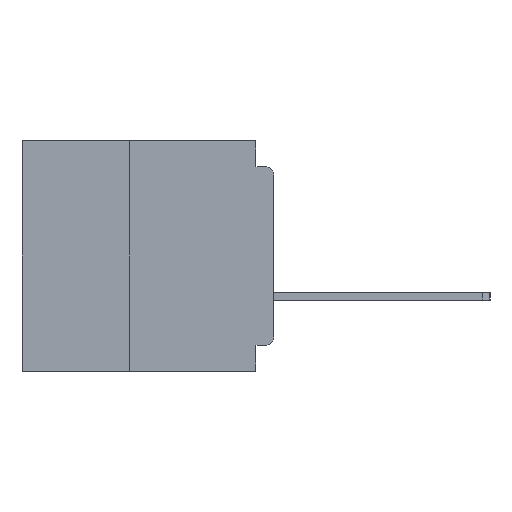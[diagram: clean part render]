
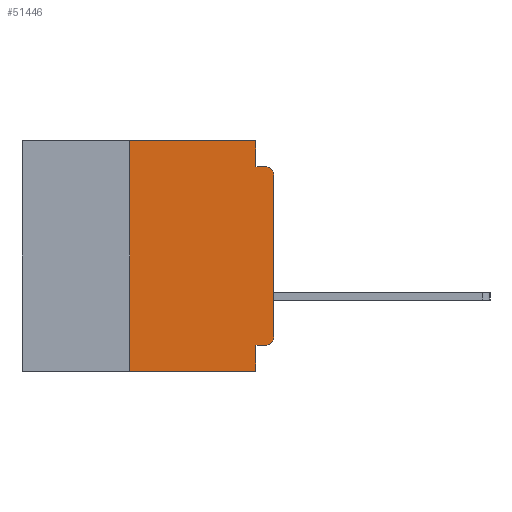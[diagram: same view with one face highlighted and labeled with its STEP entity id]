
A CAD part, left-side view. The second image highlights one B-rep face of the part: STEP entity #51446.
In plain terms, the highlighted planar face has unit normal (-1, 0, 0).
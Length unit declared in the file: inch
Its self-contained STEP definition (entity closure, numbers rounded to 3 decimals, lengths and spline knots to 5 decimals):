
#153 = FACE_OUTER_BOUND ( 'NONE', #14026, .T. ) ;
#730 = EDGE_CURVE ( 'NONE', #28737, #27394, #836, .T. ) ;
#836 = LINE ( 'NONE', #14159, #27034 ) ;
#1958 = EDGE_CURVE ( 'NONE', #6990, #15232, #45787, .T. ) ;
#3212 = CARTESIAN_POINT ( 'NONE',  ( 0., 0.437, 0. ) ) ;
#4133 = CARTESIAN_POINT ( 'NONE',  ( 0., 0.031, -0.355 ) ) ;
#5582 = ORIENTED_EDGE ( 'NONE', *, *, #59781, .F. ) ;
#5728 = LINE ( 'NONE', #22024, #30328 ) ;
#6990 = VERTEX_POINT ( 'NONE', #26731 ) ;
#7189 = AXIS2_PLACEMENT_3D ( 'NONE', #3212, #13134, #47173 ) ;
#8165 = PLANE ( 'NONE',  #7189 ) ;
#8986 = CARTESIAN_POINT ( 'NONE',  ( 0., 0.25, 0. ) ) ;
#9004 = CARTESIAN_POINT ( 'NONE',  ( 0., 0.031, 0. ) ) ;
#9005 = CARTESIAN_POINT ( 'NONE',  ( 0., 0.25, -0.4 ) ) ;
#9928 = LINE ( 'NONE', #20241, #60146 ) ;
#10337 = CIRCLE ( 'NONE', #11037, 0.015 ) ;
#11037 = AXIS2_PLACEMENT_3D ( 'NONE', #41178, #11949, #46035 ) ;
#11949 = DIRECTION ( 'NONE',  ( -1., 0., 0. ) ) ;
#13134 = DIRECTION ( 'NONE',  ( 1., 0., 0. ) ) ;
#13629 = DIRECTION ( 'NONE',  ( 0., 0., -1. ) ) ;
#14026 = EDGE_LOOP ( 'NONE', ( #23141, #17869, #46385, #5582, #19569, #17228, #19658, #22345, #46740, #44199 ) ) ;
#14159 = CARTESIAN_POINT ( 'NONE',  ( 0., 0.031, -0.4 ) ) ;
#14546 = CARTESIAN_POINT ( 'NONE',  ( 0., 0.015, -0.045 ) ) ;
#15232 = VERTEX_POINT ( 'NONE', #26761 ) ;
#15936 = CARTESIAN_POINT ( 'NONE',  ( 0., 0., -0.355 ) ) ;
#17228 = ORIENTED_EDGE ( 'NONE', *, *, #47877, .F. ) ;
#17869 = ORIENTED_EDGE ( 'NONE', *, *, #34002, .T. ) ;
#18106 = EDGE_CURVE ( 'NONE', #44121, #28737, #50356, .T. ) ;
#18987 = EDGE_CURVE ( 'NONE', #44121, #6990, #61621, .T. ) ;
#19569 = ORIENTED_EDGE ( 'NONE', *, *, #21170, .F. ) ;
#19658 = ORIENTED_EDGE ( 'NONE', *, *, #24524, .T. ) ;
#20241 = CARTESIAN_POINT ( 'NONE',  ( 0., 0.25, -0.4 ) ) ;
#21170 = EDGE_CURVE ( 'NONE', #31623, #36889, #34889, .T. ) ;
#21726 = CARTESIAN_POINT ( 'NONE',  ( 0., 0., -0.045 ) ) ;
#21965 = VECTOR ( 'NONE', #40510, 39.37008 ) ;
#22024 = CARTESIAN_POINT ( 'NONE',  ( 0., 0.031, 0. ) ) ;
#22345 = ORIENTED_EDGE ( 'NONE', *, *, #730, .F. ) ;
#23060 = VECTOR ( 'NONE', #55452, 39.37008 ) ;
#23141 = ORIENTED_EDGE ( 'NONE', *, *, #1958, .T. ) ;
#23206 = VERTEX_POINT ( 'NONE', #28243 ) ;
#23985 = VECTOR ( 'NONE', #26770, 39.37008 ) ;
#24524 = EDGE_CURVE ( 'NONE', #56850, #27394, #36855, .T. ) ;
#26731 = CARTESIAN_POINT ( 'NONE',  ( 0., 0., -0.34 ) ) ;
#26761 = CARTESIAN_POINT ( 'NONE',  ( 0., 0., -0.06 ) ) ;
#26770 = DIRECTION ( 'NONE',  ( 0., -1., 0. ) ) ;
#27034 = VECTOR ( 'NONE', #13629, 39.37008 ) ;
#27394 = VERTEX_POINT ( 'NONE', #42565 ) ;
#27434 = CARTESIAN_POINT ( 'NONE',  ( 0., 0.015, -0.34 ) ) ;
#28243 = CARTESIAN_POINT ( 'NONE',  ( 0., 0.031, -0.045 ) ) ;
#28737 = VERTEX_POINT ( 'NONE', #4133 ) ;
#30328 = VECTOR ( 'NONE', #46199, 39.37008 ) ;
#31623 = VERTEX_POINT ( 'NONE', #8986 ) ;
#32284 = DIRECTION ( 'NONE',  ( 0., 0., -1. ) ) ;
#34002 = EDGE_CURVE ( 'NONE', #15232, #50399, #10337, .T. ) ;
#34889 = LINE ( 'NONE', #59780, #21965 ) ;
#36620 = EDGE_CURVE ( 'NONE', #23206, #50399, #61707, .T. ) ;
#36855 = LINE ( 'NONE', #60603, #23985 ) ;
#36889 = VERTEX_POINT ( 'NONE', #9004 ) ;
#37510 = VECTOR ( 'NONE', #49913, 39.37008 ) ;
#40510 = DIRECTION ( 'NONE',  ( 0., -1., 0. ) ) ;
#41178 = CARTESIAN_POINT ( 'NONE',  ( 0., 0.015, -0.06 ) ) ;
#42565 = CARTESIAN_POINT ( 'NONE',  ( 0., 0.031, -0.4 ) ) ;
#44121 = VERTEX_POINT ( 'NONE', #45968 ) ;
#44199 = ORIENTED_EDGE ( 'NONE', *, *, #18987, .T. ) ;
#44464 = DIRECTION ( 'NONE',  ( 0., 0., 1. ) ) ;
#45787 = LINE ( 'NONE', #45867, #60169 ) ;
#45867 = CARTESIAN_POINT ( 'NONE',  ( 0., 0., 0. ) ) ;
#45968 = CARTESIAN_POINT ( 'NONE',  ( 0., 0.015, -0.355 ) ) ;
#46035 = DIRECTION ( 'NONE',  ( 0., 0., -1. ) ) ;
#46199 = DIRECTION ( 'NONE',  ( 0., 0., -1. ) ) ;
#46385 = ORIENTED_EDGE ( 'NONE', *, *, #36620, .F. ) ;
#46740 = ORIENTED_EDGE ( 'NONE', *, *, #18106, .F. ) ;
#47173 = DIRECTION ( 'NONE',  ( 0., 0., -1. ) ) ;
#47877 = EDGE_CURVE ( 'NONE', #56850, #31623, #9928, .T. ) ;
#49913 = DIRECTION ( 'NONE',  ( 0., 1., 0. ) ) ;
#50356 = LINE ( 'NONE', #15936, #37510 ) ;
#50399 = VERTEX_POINT ( 'NONE', #14546 ) ;
#51446 = ADVANCED_FACE ( 'NONE', ( #153 ), #8165, .F. ) ;
#55452 = DIRECTION ( 'NONE',  ( 0., -1., 0. ) ) ;
#55605 = DIRECTION ( 'NONE',  ( 0., 0., 1. ) ) ;
#56850 = VERTEX_POINT ( 'NONE', #9005 ) ;
#58438 = AXIS2_PLACEMENT_3D ( 'NONE', #27434, #61258, #32284 ) ;
#59780 = CARTESIAN_POINT ( 'NONE',  ( 0., 0.437, 0. ) ) ;
#59781 = EDGE_CURVE ( 'NONE', #36889, #23206, #5728, .T. ) ;
#60146 = VECTOR ( 'NONE', #44464, 39.37008 ) ;
#60169 = VECTOR ( 'NONE', #55605, 39.37008 ) ;
#60603 = CARTESIAN_POINT ( 'NONE',  ( 0., 0.437, -0.4 ) ) ;
#61258 = DIRECTION ( 'NONE',  ( -1., 0., 0. ) ) ;
#61621 = CIRCLE ( 'NONE', #58438, 0.015 ) ;
#61707 = LINE ( 'NONE', #21726, #23060 ) ;
